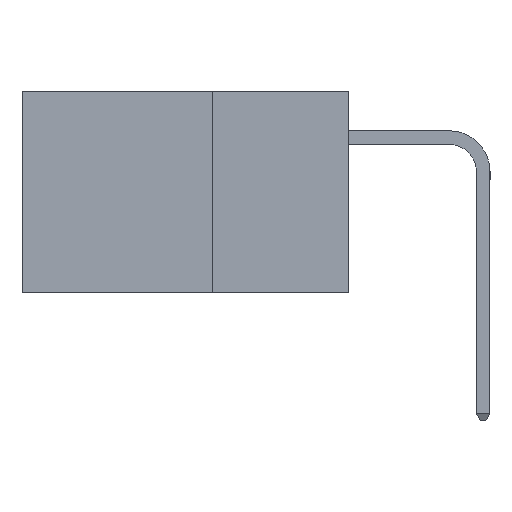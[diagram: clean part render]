
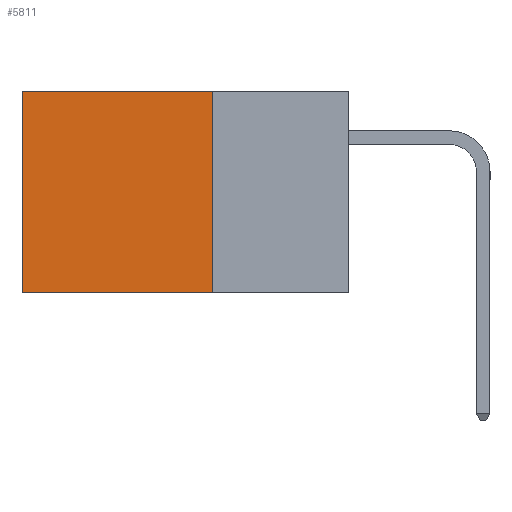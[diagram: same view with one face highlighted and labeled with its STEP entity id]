
A CAD part, left-side view. The second image highlights one B-rep face of the part: STEP entity #5811.
In plain terms, the highlighted planar face has unit normal (-1, 0, 0).
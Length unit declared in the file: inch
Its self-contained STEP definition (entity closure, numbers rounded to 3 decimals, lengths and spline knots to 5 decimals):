
#3179 = CARTESIAN_POINT ( 'NONE',  ( 0.2875, 0.25, -0.37 ) ) ;
#5053 = EDGE_CURVE ( 'NONE', #11747, #26684, #14557, .T. ) ;
#5798 = DIRECTION ( 'NONE',  ( 0., 0., -1. ) ) ;
#5811 = ADVANCED_FACE ( 'NONE', ( #13000 ), #9331, .F. ) ;
#7119 = CARTESIAN_POINT ( 'NONE',  ( 0.2875, 0.25, 0. ) ) ;
#8778 = CARTESIAN_POINT ( 'NONE',  ( 0.2875, 0.6, 0. ) ) ;
#9331 = PLANE ( 'NONE',  #39166 ) ;
#9447 = LINE ( 'NONE', #39199, #38167 ) ;
#9832 = EDGE_CURVE ( 'NONE', #26684, #10196, #31360, .T. ) ;
#10196 = VERTEX_POINT ( 'NONE', #35137 ) ;
#10430 = EDGE_CURVE ( 'NONE', #47142, #10196, #36589, .T. ) ;
#11747 = VERTEX_POINT ( 'NONE', #39539 ) ;
#11856 = ORIENTED_EDGE ( 'NONE', *, *, #10430, .F. ) ;
#12653 = EDGE_CURVE ( 'NONE', #11747, #47142, #9447, .T. ) ;
#13000 = FACE_OUTER_BOUND ( 'NONE', #23502, .T. ) ;
#14557 = LINE ( 'NONE', #28701, #37533 ) ;
#16384 = ORIENTED_EDGE ( 'NONE', *, *, #5053, .T. ) ;
#17307 = CARTESIAN_POINT ( 'NONE',  ( 0.2875, 0.25, -0.37 ) ) ;
#18060 = DIRECTION ( 'NONE',  ( 0., 1., 0. ) ) ;
#18930 = VECTOR ( 'NONE', #18060, 39.37008 ) ;
#21300 = DIRECTION ( 'NONE',  ( 0., 0., -1. ) ) ;
#23502 = EDGE_LOOP ( 'NONE', ( #27941, #11856, #25057, #16384 ) ) ;
#25057 = ORIENTED_EDGE ( 'NONE', *, *, #12653, .F. ) ;
#26684 = VERTEX_POINT ( 'NONE', #8778 ) ;
#27941 = ORIENTED_EDGE ( 'NONE', *, *, #9832, .T. ) ;
#28595 = DIRECTION ( 'NONE',  ( 1., 0., 0. ) ) ;
#28701 = CARTESIAN_POINT ( 'NONE',  ( 0.2875, 0.25, 0. ) ) ;
#29202 = DIRECTION ( 'NONE',  ( 0., 1., 0. ) ) ;
#31360 = LINE ( 'NONE', #46230, #34433 ) ;
#34433 = VECTOR ( 'NONE', #39390, 39.37008 ) ;
#35137 = CARTESIAN_POINT ( 'NONE',  ( 0.2875, 0.6, -0.37 ) ) ;
#36589 = LINE ( 'NONE', #3179, #18930 ) ;
#37533 = VECTOR ( 'NONE', #29202, 39.37008 ) ;
#38167 = VECTOR ( 'NONE', #5798, 39.37008 ) ;
#39166 = AXIS2_PLACEMENT_3D ( 'NONE', #7119, #28595, #21300 ) ;
#39199 = CARTESIAN_POINT ( 'NONE',  ( 0.2875, 0.25, 0. ) ) ;
#39390 = DIRECTION ( 'NONE',  ( 0., 0., -1. ) ) ;
#39539 = CARTESIAN_POINT ( 'NONE',  ( 0.2875, 0.25, 0. ) ) ;
#46230 = CARTESIAN_POINT ( 'NONE',  ( 0.2875, 0.6, 0. ) ) ;
#47142 = VERTEX_POINT ( 'NONE', #17307 ) ;
